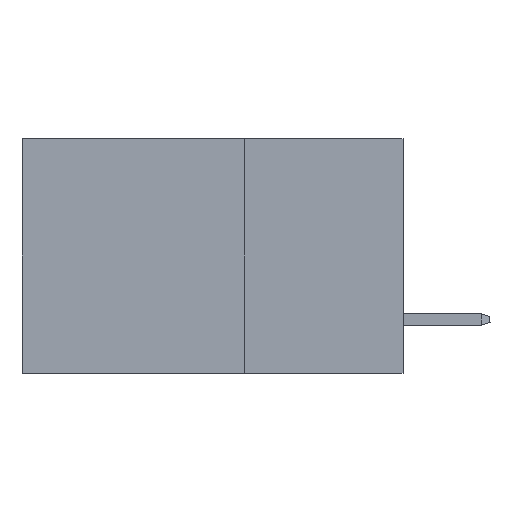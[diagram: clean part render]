
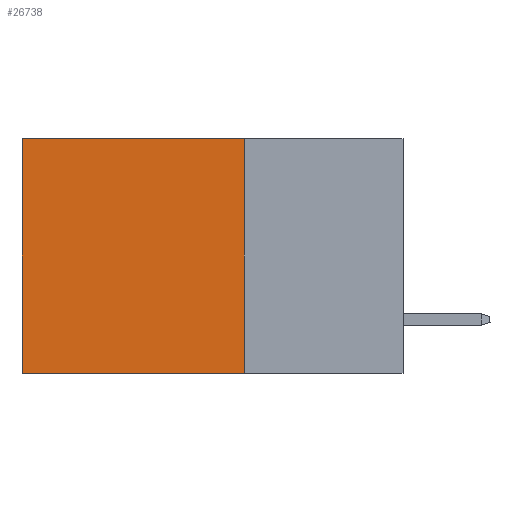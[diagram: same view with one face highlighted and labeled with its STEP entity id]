
A CAD part, left-side view. The second image highlights one B-rep face of the part: STEP entity #26738.
In plain terms, the highlighted planar face has unit normal (-1, 0, 0).
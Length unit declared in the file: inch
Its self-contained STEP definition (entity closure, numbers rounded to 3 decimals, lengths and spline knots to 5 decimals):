
#2990 = VECTOR ( 'NONE', #6127, 39.37008 ) ;
#4133 = CARTESIAN_POINT ( 'NONE',  ( 0.2875, 0.25, 0. ) ) ;
#5357 = DIRECTION ( 'NONE',  ( 0., 0., -1. ) ) ;
#5796 = VECTOR ( 'NONE', #5357, 39.37008 ) ;
#6127 = DIRECTION ( 'NONE',  ( 0., 0., -1. ) ) ;
#7004 = ORIENTED_EDGE ( 'NONE', *, *, #7471, .F. ) ;
#7247 = DIRECTION ( 'NONE',  ( 0., 1., 0. ) ) ;
#7423 = LINE ( 'NONE', #4133, #2990 ) ;
#7471 = EDGE_CURVE ( 'NONE', #24175, #17926, #7423, .T. ) ;
#7844 = VECTOR ( 'NONE', #7247, 39.37008 ) ;
#8602 = ORIENTED_EDGE ( 'NONE', *, *, #17210, .F. ) ;
#9474 = LINE ( 'NONE', #11738, #5796 ) ;
#11645 = EDGE_CURVE ( 'NONE', #26686, #13221, #9474, .T. ) ;
#11738 = CARTESIAN_POINT ( 'NONE',  ( 0.2875, 0.6, 0. ) ) ;
#12198 = CARTESIAN_POINT ( 'NONE',  ( 0.2875, 0.6, -0.37 ) ) ;
#12398 = ORIENTED_EDGE ( 'NONE', *, *, #11645, .T. ) ;
#13221 = VERTEX_POINT ( 'NONE', #12198 ) ;
#13299 = CARTESIAN_POINT ( 'NONE',  ( 0.2875, 0.25, 0. ) ) ;
#13615 = EDGE_CURVE ( 'NONE', #24175, #26686, #20488, .T. ) ;
#13872 = CARTESIAN_POINT ( 'NONE',  ( 0.2875, 0.25, -0.37 ) ) ;
#15957 = CARTESIAN_POINT ( 'NONE',  ( 0.2875, 0.25, 0. ) ) ;
#16963 = CARTESIAN_POINT ( 'NONE',  ( 0.2875, 0.25, -0.37 ) ) ;
#17210 = EDGE_CURVE ( 'NONE', #17926, #13221, #19981, .T. ) ;
#17926 = VERTEX_POINT ( 'NONE', #16963 ) ;
#18216 = DIRECTION ( 'NONE',  ( 0., 1., 0. ) ) ;
#18802 = AXIS2_PLACEMENT_3D ( 'NONE', #23596, #19488, #21058 ) ;
#19488 = DIRECTION ( 'NONE',  ( 1., 0., 0. ) ) ;
#19981 = LINE ( 'NONE', #13872, #7844 ) ;
#20358 = VECTOR ( 'NONE', #18216, 39.37008 ) ;
#20488 = LINE ( 'NONE', #15957, #20358 ) ;
#21032 = ORIENTED_EDGE ( 'NONE', *, *, #13615, .T. ) ;
#21058 = DIRECTION ( 'NONE',  ( 0., 0., -1. ) ) ;
#22642 = EDGE_LOOP ( 'NONE', ( #12398, #8602, #7004, #21032 ) ) ;
#23318 = FACE_OUTER_BOUND ( 'NONE', #22642, .T. ) ;
#23596 = CARTESIAN_POINT ( 'NONE',  ( 0.2875, 0.25, 0. ) ) ;
#24175 = VERTEX_POINT ( 'NONE', #13299 ) ;
#26000 = PLANE ( 'NONE',  #18802 ) ;
#26686 = VERTEX_POINT ( 'NONE', #27422 ) ;
#26738 = ADVANCED_FACE ( 'NONE', ( #23318 ), #26000, .F. ) ;
#27422 = CARTESIAN_POINT ( 'NONE',  ( 0.2875, 0.6, 0. ) ) ;
